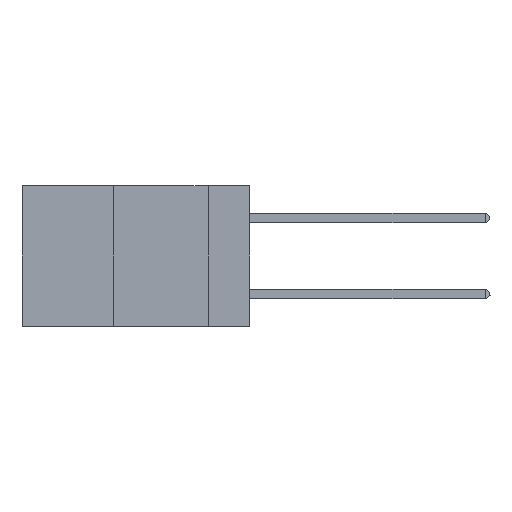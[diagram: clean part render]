
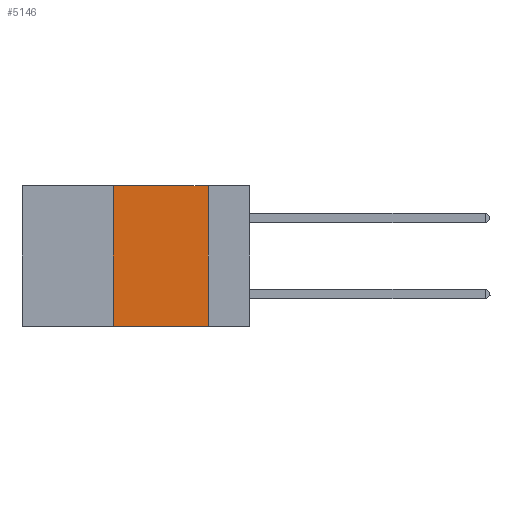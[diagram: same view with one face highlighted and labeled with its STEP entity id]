
A CAD part, left-side view. The second image highlights one B-rep face of the part: STEP entity #5146.
In plain terms, the highlighted planar face has unit normal (-1, 0, 0).
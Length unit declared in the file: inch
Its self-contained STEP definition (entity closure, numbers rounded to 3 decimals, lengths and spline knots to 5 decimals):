
#109 = CARTESIAN_POINT ( 'NONE',  ( 0., 0.6, 0. ) ) ;
#679 = VERTEX_POINT ( 'NONE', #4919 ) ;
#713 = DIRECTION ( 'NONE',  ( 1., 0., 0. ) ) ;
#1060 = CARTESIAN_POINT ( 'NONE',  ( 0., 0.36, 0. ) ) ;
#1421 = CARTESIAN_POINT ( 'NONE',  ( 0., 0.36, 0. ) ) ;
#1610 = DIRECTION ( 'NONE',  ( 0., 0., -1. ) ) ;
#1611 = EDGE_CURVE ( 'NONE', #5465, #7994, #4362, .T. ) ;
#1766 = VECTOR ( 'NONE', #6400, 39.37008 ) ;
#2130 = LINE ( 'NONE', #10508, #11831 ) ;
#2260 = VECTOR ( 'NONE', #10057, 39.37008 ) ;
#2521 = DIRECTION ( 'NONE',  ( 0., -1., 0. ) ) ;
#2601 = DIRECTION ( 'NONE',  ( 0., 0., -1. ) ) ;
#2776 = VERTEX_POINT ( 'NONE', #4085 ) ;
#3075 = CARTESIAN_POINT ( 'NONE',  ( 0., 0.6, 0. ) ) ;
#3377 = ORIENTED_EDGE ( 'NONE', *, *, #4642, .F. ) ;
#3393 = VECTOR ( 'NONE', #1610, 39.37008 ) ;
#3802 = ORIENTED_EDGE ( 'NONE', *, *, #1611, .F. ) ;
#4085 = CARTESIAN_POINT ( 'NONE',  ( 0., 0.36, -0.37 ) ) ;
#4362 = LINE ( 'NONE', #3075, #1766 ) ;
#4642 = EDGE_CURVE ( 'NONE', #7994, #679, #8493, .T. ) ;
#4853 = AXIS2_PLACEMENT_3D ( 'NONE', #109, #713, #2601 ) ;
#4919 = CARTESIAN_POINT ( 'NONE',  ( 0., 0.11, -0.37 ) ) ;
#5070 = EDGE_CURVE ( 'NONE', #2776, #679, #2130, .T. ) ;
#5146 = ADVANCED_FACE ( 'NONE', ( #11283 ), #5922, .F. ) ;
#5465 = VERTEX_POINT ( 'NONE', #1060 ) ;
#5922 = PLANE ( 'NONE',  #4853 ) ;
#6400 = DIRECTION ( 'NONE',  ( 0., -1., 0. ) ) ;
#7398 = LINE ( 'NONE', #1421, #2260 ) ;
#7994 = VERTEX_POINT ( 'NONE', #9088 ) ;
#8493 = LINE ( 'NONE', #11943, #3393 ) ;
#9088 = CARTESIAN_POINT ( 'NONE',  ( 0., 0.11, 0. ) ) ;
#9499 = EDGE_LOOP ( 'NONE', ( #3377, #3802, #9767, #12216 ) ) ;
#9767 = ORIENTED_EDGE ( 'NONE', *, *, #11152, .F. ) ;
#10057 = DIRECTION ( 'NONE',  ( 0., 0., 1. ) ) ;
#10508 = CARTESIAN_POINT ( 'NONE',  ( 0., 0.6, -0.37 ) ) ;
#11152 = EDGE_CURVE ( 'NONE', #2776, #5465, #7398, .T. ) ;
#11283 = FACE_OUTER_BOUND ( 'NONE', #9499, .T. ) ;
#11831 = VECTOR ( 'NONE', #2521, 39.37008 ) ;
#11943 = CARTESIAN_POINT ( 'NONE',  ( 0., 0.11, 0. ) ) ;
#12216 = ORIENTED_EDGE ( 'NONE', *, *, #5070, .T. ) ;
